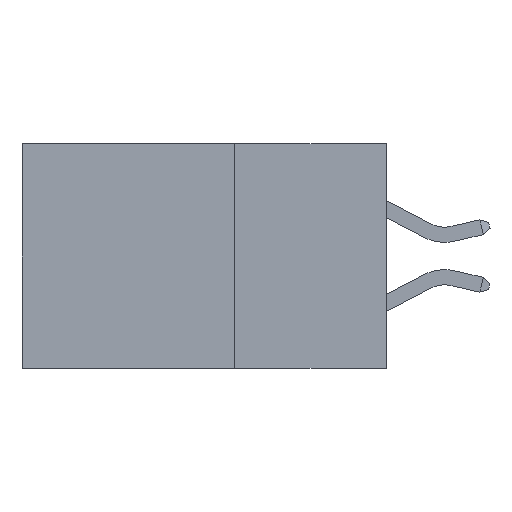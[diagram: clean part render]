
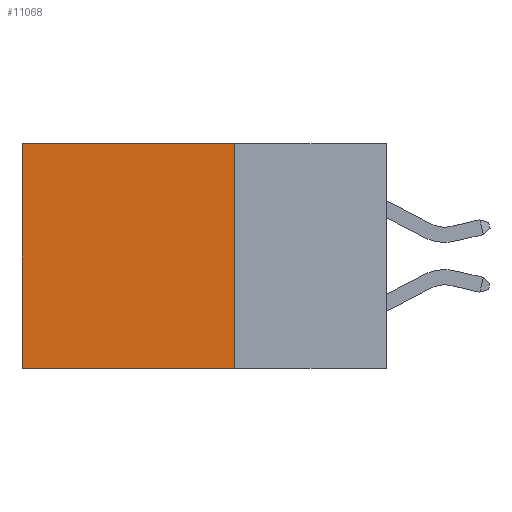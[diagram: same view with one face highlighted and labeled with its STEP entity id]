
A CAD part, left-side view. The second image highlights one B-rep face of the part: STEP entity #11068.
In plain terms, the highlighted planar face has unit normal (-1, 0, 0).
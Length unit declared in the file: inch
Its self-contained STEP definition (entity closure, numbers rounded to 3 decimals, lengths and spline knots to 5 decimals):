
#9 = DIRECTION ( 'NONE',  ( 1., 0., 0. ) ) ;
#354 = AXIS2_PLACEMENT_3D ( 'NONE', #980, #9, #8517 ) ;
#461 = VERTEX_POINT ( 'NONE', #4420 ) ;
#717 = CARTESIAN_POINT ( 'NONE',  ( 0.2615, 0.25, -0.37 ) ) ;
#895 = VECTOR ( 'NONE', #8927, 39.37008 ) ;
#980 = CARTESIAN_POINT ( 'NONE',  ( 0.2615, 0.25, -0.37 ) ) ;
#1057 = CARTESIAN_POINT ( 'NONE',  ( 0.2615, 0.25, -0.37 ) ) ;
#1088 = VECTOR ( 'NONE', #11806, 39.37008 ) ;
#2293 = ORIENTED_EDGE ( 'NONE', *, *, #9295, .F. ) ;
#3599 = CARTESIAN_POINT ( 'NONE',  ( 0.2615, 0.25, -0.37 ) ) ;
#3907 = DIRECTION ( 'NONE',  ( 0., 0., -1. ) ) ;
#4420 = CARTESIAN_POINT ( 'NONE',  ( 0.2615, 0.25, 0. ) ) ;
#4425 = DIRECTION ( 'NONE',  ( 0., 1., 0. ) ) ;
#5220 = CARTESIAN_POINT ( 'NONE',  ( 0.2615, 0.6, -0.37 ) ) ;
#5480 = PLANE ( 'NONE',  #354 ) ;
#5760 = LINE ( 'NONE', #717, #8144 ) ;
#6034 = EDGE_CURVE ( 'NONE', #461, #6524, #10942, .T. ) ;
#6225 = CARTESIAN_POINT ( 'NONE',  ( 0.2615, 0.25, 0. ) ) ;
#6462 = ORIENTED_EDGE ( 'NONE', *, *, #6034, .T. ) ;
#6524 = VERTEX_POINT ( 'NONE', #11966 ) ;
#6567 = CARTESIAN_POINT ( 'NONE',  ( 0.2615, 0.6, -0.37 ) ) ;
#6568 = VERTEX_POINT ( 'NONE', #6567 ) ;
#6949 = VECTOR ( 'NONE', #3907, 39.37008 ) ;
#7541 = ORIENTED_EDGE ( 'NONE', *, *, #8985, .T. ) ;
#8089 = ORIENTED_EDGE ( 'NONE', *, *, #11803, .F. ) ;
#8144 = VECTOR ( 'NONE', #4425, 39.37008 ) ;
#8517 = DIRECTION ( 'NONE',  ( 0., 0., -1. ) ) ;
#8625 = LINE ( 'NONE', #5220, #895 ) ;
#8927 = DIRECTION ( 'NONE',  ( 0., 0., -1. ) ) ;
#8985 = EDGE_CURVE ( 'NONE', #6524, #6568, #8625, .T. ) ;
#9295 = EDGE_CURVE ( 'NONE', #461, #9495, #10416, .T. ) ;
#9423 = FACE_OUTER_BOUND ( 'NONE', #10132, .T. ) ;
#9495 = VERTEX_POINT ( 'NONE', #3599 ) ;
#10132 = EDGE_LOOP ( 'NONE', ( #7541, #8089, #2293, #6462 ) ) ;
#10416 = LINE ( 'NONE', #1057, #6949 ) ;
#10942 = LINE ( 'NONE', #6225, #1088 ) ;
#11068 = ADVANCED_FACE ( 'NONE', ( #9423 ), #5480, .F. ) ;
#11803 = EDGE_CURVE ( 'NONE', #9495, #6568, #5760, .T. ) ;
#11806 = DIRECTION ( 'NONE',  ( 0., 1., 0. ) ) ;
#11966 = CARTESIAN_POINT ( 'NONE',  ( 0.2615, 0.6, 0. ) ) ;
